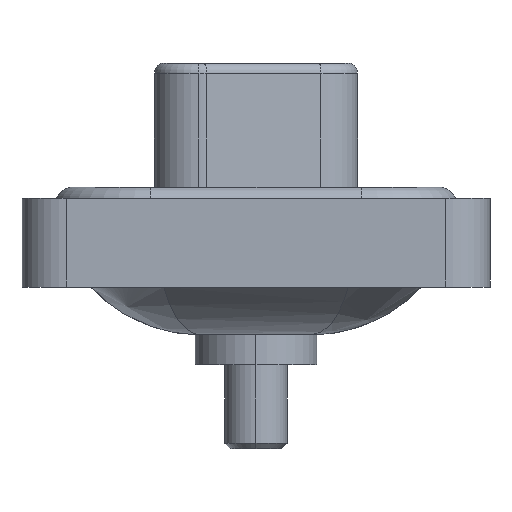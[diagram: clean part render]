
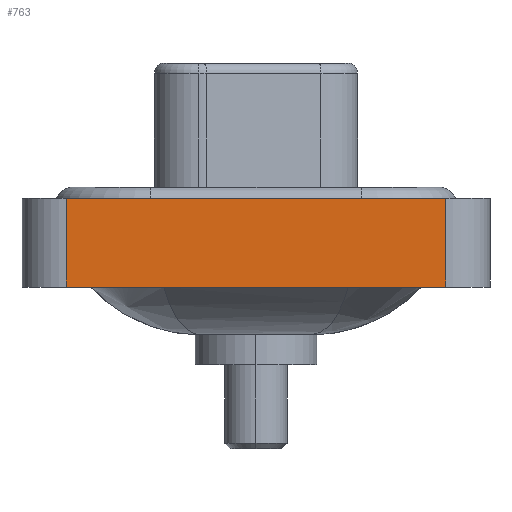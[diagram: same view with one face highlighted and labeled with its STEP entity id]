
A CAD part, left-side view. The second image highlights one B-rep face of the part: STEP entity #763.
In plain terms, the highlighted planar face has unit normal (-1, 0, 0).
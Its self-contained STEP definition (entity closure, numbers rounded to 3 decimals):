
#507 = VERTEX_POINT ( 'NONE', #4728 ) ;
#763 = ADVANCED_FACE ( 'NONE', ( #1669 ), #16335, .T. ) ;
#786 = CARTESIAN_POINT ( 'NONE',  ( -7.3, 8.55, 0.4 ) ) ;
#1669 = FACE_OUTER_BOUND ( 'NONE', #10240, .T. ) ;
#2484 = CARTESIAN_POINT ( 'NONE',  ( -7.3, 8.55, -3.6 ) ) ;
#2490 = EDGE_CURVE ( 'NONE', #10340, #6695, #17611, .T. ) ;
#2818 = VECTOR ( 'NONE', #4320, 1000. ) ;
#2830 = DIRECTION ( 'NONE',  ( 0., 0., 1. ) ) ;
#3139 = EDGE_CURVE ( 'NONE', #507, #9333, #8848, .T. ) ;
#3373 = VECTOR ( 'NONE', #2830, 1000. ) ;
#4320 = DIRECTION ( 'NONE',  ( 0., -1., 0. ) ) ;
#4490 = CARTESIAN_POINT ( 'NONE',  ( -7.3, -8.55, -3.6 ) ) ;
#4728 = CARTESIAN_POINT ( 'NONE',  ( -7.3, 8.55, -3.6 ) ) ;
#5573 = DIRECTION ( 'NONE',  ( 0., 0., 1. ) ) ;
#5735 = DIRECTION ( 'NONE',  ( -1., 0., 0. ) ) ;
#6195 = AXIS2_PLACEMENT_3D ( 'NONE', #11717, #5735, #11626 ) ;
#6271 = ORIENTED_EDGE ( 'NONE', *, *, #3139, .T. ) ;
#6653 = CARTESIAN_POINT ( 'NONE',  ( -7.3, -8.55, -3.6 ) ) ;
#6695 = VERTEX_POINT ( 'NONE', #10161 ) ;
#6751 = ORIENTED_EDGE ( 'NONE', *, *, #2490, .F. ) ;
#8848 = LINE ( 'NONE', #17509, #12924 ) ;
#9333 = VERTEX_POINT ( 'NONE', #6653 ) ;
#10161 = CARTESIAN_POINT ( 'NONE',  ( -7.3, -8.55, 0.4 ) ) ;
#10240 = EDGE_LOOP ( 'NONE', ( #11481, #6751, #14819, #6271 ) ) ;
#10340 = VERTEX_POINT ( 'NONE', #786 ) ;
#11481 = ORIENTED_EDGE ( 'NONE', *, *, #12275, .T. ) ;
#11626 = DIRECTION ( 'NONE',  ( 0., 0., 1. ) ) ;
#11717 = CARTESIAN_POINT ( 'NONE',  ( -7.3, -8.55, -3.6 ) ) ;
#11804 = LINE ( 'NONE', #4490, #3373 ) ;
#12275 = EDGE_CURVE ( 'NONE', #9333, #6695, #11804, .T. ) ;
#12924 = VECTOR ( 'NONE', #13174, 1000. ) ;
#13174 = DIRECTION ( 'NONE',  ( 0., -1., 0. ) ) ;
#14615 = EDGE_CURVE ( 'NONE', #507, #10340, #18763, .T. ) ;
#14819 = ORIENTED_EDGE ( 'NONE', *, *, #14615, .F. ) ;
#16335 = PLANE ( 'NONE',  #6195 ) ;
#17043 = VECTOR ( 'NONE', #5573, 1000. ) ;
#17509 = CARTESIAN_POINT ( 'NONE',  ( -7.3, -8.55, -3.6 ) ) ;
#17611 = LINE ( 'NONE', #18854, #2818 ) ;
#18763 = LINE ( 'NONE', #2484, #17043 ) ;
#18854 = CARTESIAN_POINT ( 'NONE',  ( -7.3, -8.55, 0.4 ) ) ;
